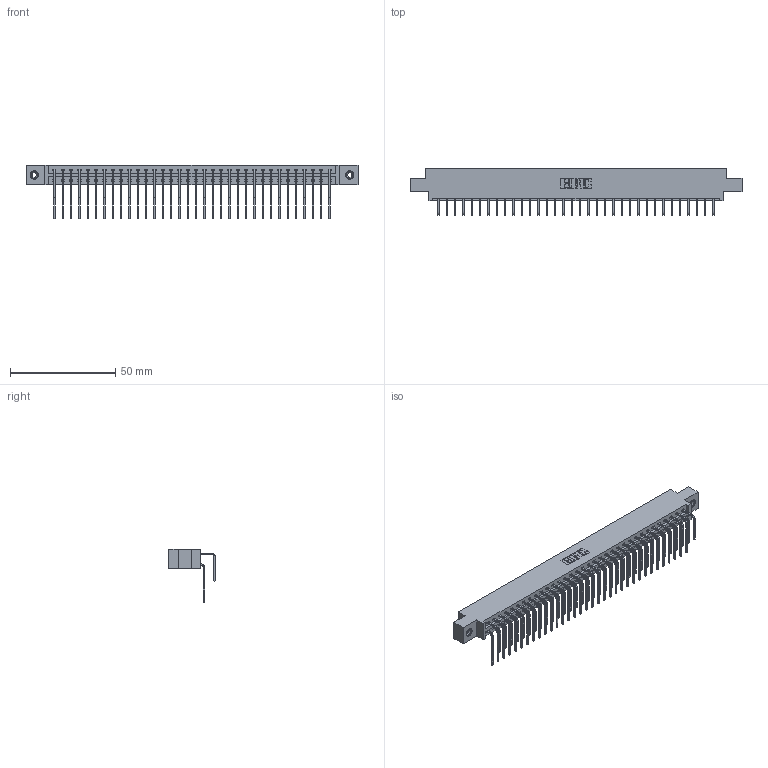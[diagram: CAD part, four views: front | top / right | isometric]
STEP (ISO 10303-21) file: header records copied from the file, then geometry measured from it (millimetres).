
FILE_DESCRIPTION (( 'STEP AP203' ), '1' );
FILE_NAME ('337-068-558-808.STEP', '2019-10-12T02:40:51', ( '' ), ( '' ), 'SwSTEP 2.0', 'SolidWorks 2016', '' );
FILE_SCHEMA (( 'CONFIG_CONTROL_DESIGN' ));
Length unit declared in the file: inch
Products named in the file (5): 345-292-001_558 Tail - 2; 337-068-558-808; 345-292-001_558 559 Tail - 1; 345-250-001_345-250-003-102; 337 Part_0.170 Offset - 0.156 Dia-TI
Assembly tree (71 placements, depth 2):
  337-068-558-808
    337 Part_0.170 Offset - 0.156 Dia-TI
    345-292-001_558 559 Tail - 1  x34
    345-292-001_558 Tail - 2  x34
    345-250-001_345-250-003-102  x2
Bounding box: 157.73 x 22.17 x 25.53 mm (x, y, z)
Volume: 16785 mm3; surface area: 20999.2 mm2
Topology: 71 solids, 71 shells, 3986 faces, 11815 edges, 7778 vertices
Faces by surface type: plane 2826, cylinder 1144, cone 12, torus 4
Entity records: 30498 total; most frequent: CARTESIAN_POINT 5172, ORIENTED_EDGE 5050, DIRECTION 4427, EDGE_CURVE 2525, VECTOR 2337, LINE 2337, VERTEX_POINT 1676, AXIS2_PLACEMENT_3D 1045
